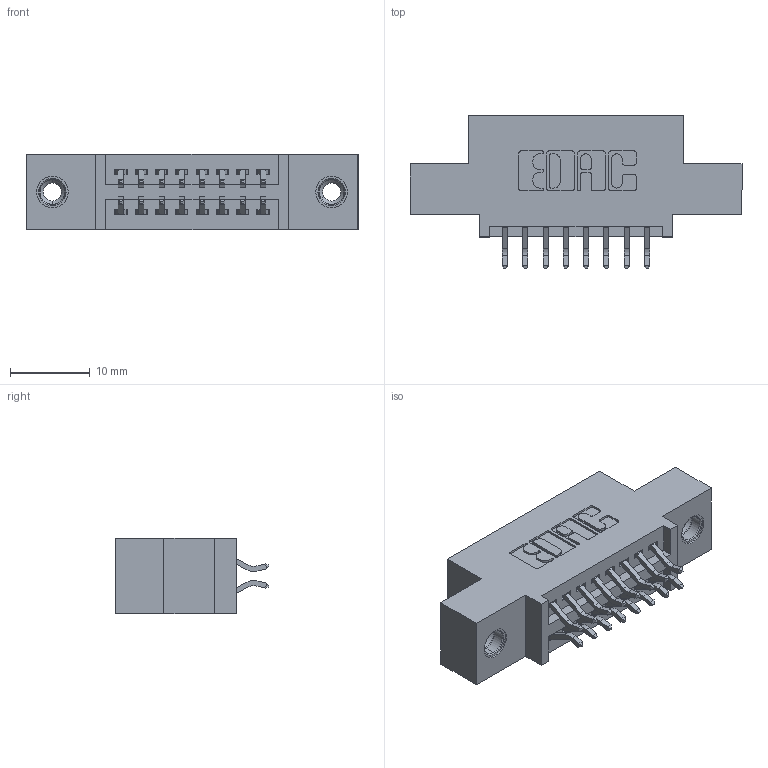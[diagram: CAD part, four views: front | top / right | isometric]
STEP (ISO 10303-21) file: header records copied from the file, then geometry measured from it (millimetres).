
FILE_DESCRIPTION (( 'STEP AP203' ), '1' );
FILE_NAME ('345-016-556-508.STEP', '2018-08-19T01:06:59', ( '' ), ( '' ), 'SwSTEP 2.0', 'SolidWorks 2016', '' );
FILE_SCHEMA (( 'CONFIG_CONTROL_DESIGN' ));
Length unit declared in the file: inch
Products named in the file (4): 345 Part_0.110 Offset - 0.156 Dia-TI; 345-292-001_556 Tail; 345-250-001_345-250-003-102; 345-016-556-508
Assembly tree (19 placements, depth 2):
  345-016-556-508
    345 Part_0.110 Offset - 0.156 Dia-TI
    345-292-001_556 Tail  x16
    345-250-001_345-250-003-102  x2
Bounding box: 41.53 x 19.24 x 9.4 mm (x, y, z)
Volume: 3638.1 mm3; surface area: 4811.4 mm2
Topology: 19 solids, 19 shells, 1086 faces, 3161 edges, 2078 vertices
Faces by surface type: plane 708, cylinder 362, cone 12, torus 4
Entity records: 12392 total; most frequent: CARTESIAN_POINT 2107, ORIENTED_EDGE 2022, DIRECTION 1913, EDGE_CURVE 1011, LINE 819, VECTOR 819, VERTEX_POINT 668, AXIS2_PLACEMENT_3D 547
